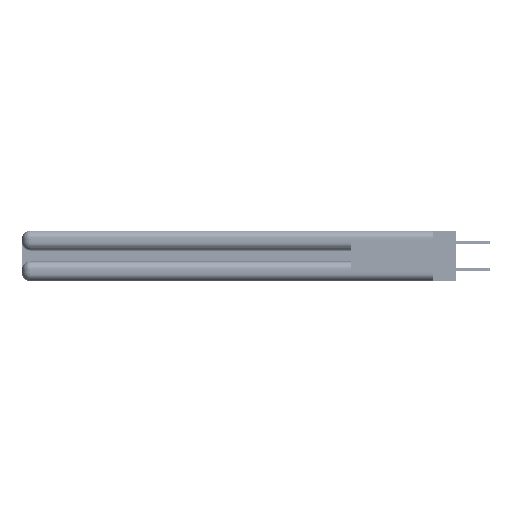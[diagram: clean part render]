
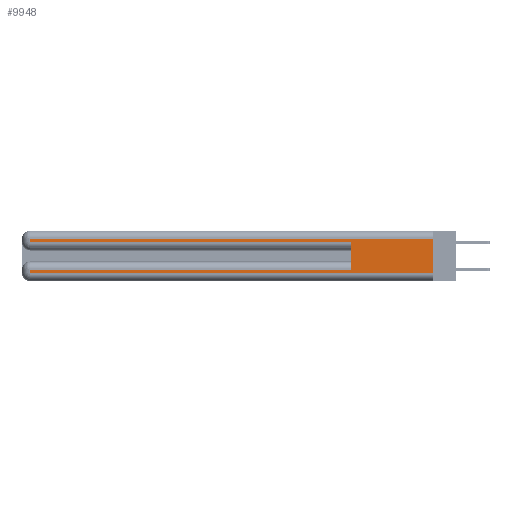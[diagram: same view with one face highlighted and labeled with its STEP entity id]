
A CAD part, left-side view. The second image highlights one B-rep face of the part: STEP entity #9948.
In plain terms, the highlighted planar face has unit normal (-1, 0, 0).
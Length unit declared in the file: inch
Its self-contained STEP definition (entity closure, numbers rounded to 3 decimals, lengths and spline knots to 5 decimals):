
#286 = ORIENTED_EDGE ( 'NONE', *, *, #37169, .T. ) ;
#412 = VECTOR ( 'NONE', #46377, 39.37008 ) ;
#1094 = DIRECTION ( 'NONE',  ( 1., 0., 0. ) ) ;
#1591 = CARTESIAN_POINT ( 'NONE',  ( 0., 0., 0.37 ) ) ;
#3190 = CARTESIAN_POINT ( 'NONE',  ( 0., 2.94, 0.37 ) ) ;
#3255 = ORIENTED_EDGE ( 'NONE', *, *, #29998, .T. ) ;
#3535 = CARTESIAN_POINT ( 'NONE',  ( 0., 2.94, 0.285 ) ) ;
#3861 = CARTESIAN_POINT ( 'NONE',  ( 0., 0., 0.085 ) ) ;
#4062 = VECTOR ( 'NONE', #37631, 39.37008 ) ;
#7584 = ORIENTED_EDGE ( 'NONE', *, *, #8847, .T. ) ;
#7958 = LINE ( 'NONE', #36682, #31715 ) ;
#8847 = EDGE_CURVE ( 'NONE', #37070, #14645, #28045, .T. ) ;
#8951 = PLANE ( 'NONE',  #31337 ) ;
#9296 = VECTOR ( 'NONE', #22183, 39.37008 ) ;
#9948 = ADVANCED_FACE ( 'NONE', ( #46164 ), #8951, .F. ) ;
#10979 = CARTESIAN_POINT ( 'NONE',  ( 0., 0.6, 0.145 ) ) ;
#11350 = DIRECTION ( 'NONE',  ( 0., 0., -1. ) ) ;
#12010 = ORIENTED_EDGE ( 'NONE', *, *, #24190, .T. ) ;
#13478 = ORIENTED_EDGE ( 'NONE', *, *, #31871, .T. ) ;
#13802 = VERTEX_POINT ( 'NONE', #3535 ) ;
#13860 = CARTESIAN_POINT ( 'NONE',  ( 0., 2.94, 0.31 ) ) ;
#14070 = DIRECTION ( 'NONE',  ( 0., 0., -1. ) ) ;
#14645 = VERTEX_POINT ( 'NONE', #35206 ) ;
#17138 = VERTEX_POINT ( 'NONE', #25194 ) ;
#18586 = LINE ( 'NONE', #37368, #45821 ) ;
#19085 = LINE ( 'NONE', #10979, #9296 ) ;
#20788 = CARTESIAN_POINT ( 'NONE',  ( 0., 0., 0.06 ) ) ;
#22183 = DIRECTION ( 'NONE',  ( 0., 0., 1. ) ) ;
#24190 = EDGE_CURVE ( 'NONE', #14645, #25774, #34610, .T. ) ;
#24243 = EDGE_CURVE ( 'NONE', #30346, #13802, #7958, .T. ) ;
#25194 = CARTESIAN_POINT ( 'NONE',  ( 0., 0., 0.31 ) ) ;
#25774 = VERTEX_POINT ( 'NONE', #37721 ) ;
#26497 = VECTOR ( 'NONE', #14070, 39.37008 ) ;
#26566 = ORIENTED_EDGE ( 'NONE', *, *, #43072, .F. ) ;
#26860 = VECTOR ( 'NONE', #44381, 39.37008 ) ;
#27049 = DIRECTION ( 'NONE',  ( 0., 0., -1. ) ) ;
#28045 = LINE ( 'NONE', #3861, #26860 ) ;
#28880 = VERTEX_POINT ( 'NONE', #38036 ) ;
#29282 = CARTESIAN_POINT ( 'NONE',  ( 0., 0.6, 0.285 ) ) ;
#29418 = EDGE_CURVE ( 'NONE', #17138, #28880, #18586, .T. ) ;
#29625 = EDGE_LOOP ( 'NONE', ( #38571, #3255, #32451, #286, #26566, #7584, #12010, #13478 ) ) ;
#29992 = LINE ( 'NONE', #20788, #412 ) ;
#29998 = EDGE_CURVE ( 'NONE', #17138, #30346, #33591, .T. ) ;
#30346 = VERTEX_POINT ( 'NONE', #13860 ) ;
#31337 = AXIS2_PLACEMENT_3D ( 'NONE', #1591, #1094, #27049 ) ;
#31684 = CARTESIAN_POINT ( 'NONE',  ( 0., 0.6, 0.085 ) ) ;
#31715 = VECTOR ( 'NONE', #43515, 39.37008 ) ;
#31871 = EDGE_CURVE ( 'NONE', #25774, #28880, #29992, .T. ) ;
#32451 = ORIENTED_EDGE ( 'NONE', *, *, #24243, .T. ) ;
#33591 = LINE ( 'NONE', #33885, #4062 ) ;
#33885 = CARTESIAN_POINT ( 'NONE',  ( 0., 0., 0.31 ) ) ;
#34610 = LINE ( 'NONE', #3190, #26497 ) ;
#35206 = CARTESIAN_POINT ( 'NONE',  ( 0., 2.94, 0.085 ) ) ;
#36091 = LINE ( 'NONE', #39269, #40720 ) ;
#36682 = CARTESIAN_POINT ( 'NONE',  ( 0., 2.94, 0.37 ) ) ;
#37070 = VERTEX_POINT ( 'NONE', #31684 ) ;
#37169 = EDGE_CURVE ( 'NONE', #13802, #46572, #36091, .T. ) ;
#37368 = CARTESIAN_POINT ( 'NONE',  ( 0., 0., 0.37 ) ) ;
#37631 = DIRECTION ( 'NONE',  ( 0., 1., 0. ) ) ;
#37721 = CARTESIAN_POINT ( 'NONE',  ( 0., 2.94, 0.06 ) ) ;
#38036 = CARTESIAN_POINT ( 'NONE',  ( 0., 0., 0.06 ) ) ;
#38571 = ORIENTED_EDGE ( 'NONE', *, *, #29418, .F. ) ;
#39269 = CARTESIAN_POINT ( 'NONE',  ( 0., 0., 0.285 ) ) ;
#40720 = VECTOR ( 'NONE', #46788, 39.37008 ) ;
#43072 = EDGE_CURVE ( 'NONE', #37070, #46572, #19085, .T. ) ;
#43515 = DIRECTION ( 'NONE',  ( 0., 0., -1. ) ) ;
#44381 = DIRECTION ( 'NONE',  ( 0., 1., 0. ) ) ;
#45821 = VECTOR ( 'NONE', #11350, 39.37008 ) ;
#46164 = FACE_OUTER_BOUND ( 'NONE', #29625, .T. ) ;
#46377 = DIRECTION ( 'NONE',  ( 0., -1., 0. ) ) ;
#46572 = VERTEX_POINT ( 'NONE', #29282 ) ;
#46788 = DIRECTION ( 'NONE',  ( 0., -1., 0. ) ) ;
